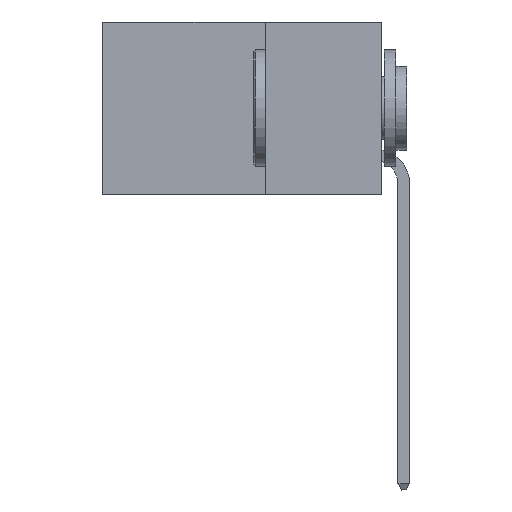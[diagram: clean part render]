
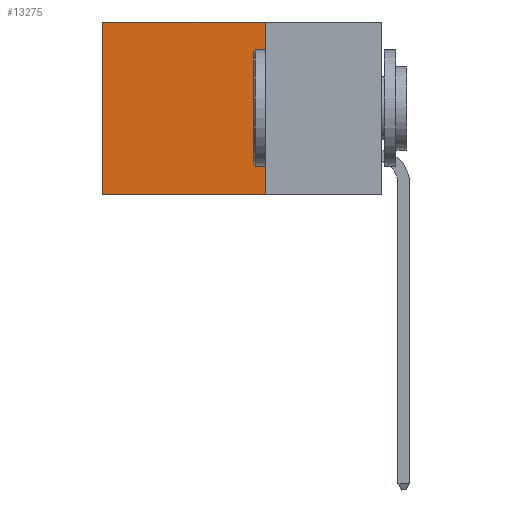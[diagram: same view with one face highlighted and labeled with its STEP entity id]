
A CAD part, left-side view. The second image highlights one B-rep face of the part: STEP entity #13275.
In plain terms, the highlighted planar face has unit normal (-1, 0, 0).
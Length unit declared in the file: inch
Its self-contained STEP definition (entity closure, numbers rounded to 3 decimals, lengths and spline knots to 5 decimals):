
#234 = DIRECTION ( 'NONE',  ( 0., 0., -1. ) ) ;
#1116 = CARTESIAN_POINT ( 'NONE',  ( 0.2875, 0.25, 0. ) ) ;
#3509 = AXIS2_PLACEMENT_3D ( 'NONE', #12520, #12021, #234 ) ;
#4520 = ORIENTED_EDGE ( 'NONE', *, *, #38850, .F. ) ;
#5057 = VERTEX_POINT ( 'NONE', #36150 ) ;
#5293 = CARTESIAN_POINT ( 'NONE',  ( 0.2875, 0.25, -0.37 ) ) ;
#5307 = VECTOR ( 'NONE', #11390, 39.37008 ) ;
#5490 = LINE ( 'NONE', #24578, #9297 ) ;
#6657 = ORIENTED_EDGE ( 'NONE', *, *, #25277, .F. ) ;
#6830 = EDGE_LOOP ( 'NONE', ( #22194, #4520, #6657, #36338 ) ) ;
#9297 = VECTOR ( 'NONE', #13358, 39.37008 ) ;
#11390 = DIRECTION ( 'NONE',  ( 0., 1., 0. ) ) ;
#12021 = DIRECTION ( 'NONE',  ( 1., 0., 0. ) ) ;
#12178 = FACE_OUTER_BOUND ( 'NONE', #6830, .T. ) ;
#12520 = CARTESIAN_POINT ( 'NONE',  ( 0.2875, 0.25, 0. ) ) ;
#13275 = ADVANCED_FACE ( 'NONE', ( #12178 ), #33258, .F. ) ;
#13325 = LINE ( 'NONE', #5293, #5307 ) ;
#13358 = DIRECTION ( 'NONE',  ( 0., 0., -1. ) ) ;
#14139 = DIRECTION ( 'NONE',  ( 0., 1., 0. ) ) ;
#14251 = VECTOR ( 'NONE', #25146, 39.37008 ) ;
#20181 = VERTEX_POINT ( 'NONE', #28641 ) ;
#21384 = LINE ( 'NONE', #26181, #26570 ) ;
#22194 = ORIENTED_EDGE ( 'NONE', *, *, #34258, .T. ) ;
#24578 = CARTESIAN_POINT ( 'NONE',  ( 0.2875, 0.6, 0. ) ) ;
#25146 = DIRECTION ( 'NONE',  ( 0., 0., -1. ) ) ;
#25277 = EDGE_CURVE ( 'NONE', #5057, #20181, #32249, .T. ) ;
#26181 = CARTESIAN_POINT ( 'NONE',  ( 0.2875, 0.25, 0. ) ) ;
#26570 = VECTOR ( 'NONE', #14139, 39.37008 ) ;
#28641 = CARTESIAN_POINT ( 'NONE',  ( 0.2875, 0.25, -0.37 ) ) ;
#30964 = EDGE_CURVE ( 'NONE', #5057, #31340, #21384, .T. ) ;
#31340 = VERTEX_POINT ( 'NONE', #36558 ) ;
#32249 = LINE ( 'NONE', #1116, #14251 ) ;
#33258 = PLANE ( 'NONE',  #3509 ) ;
#34258 = EDGE_CURVE ( 'NONE', #31340, #39076, #5490, .T. ) ;
#36150 = CARTESIAN_POINT ( 'NONE',  ( 0.2875, 0.25, 0. ) ) ;
#36186 = CARTESIAN_POINT ( 'NONE',  ( 0.2875, 0.6, -0.37 ) ) ;
#36338 = ORIENTED_EDGE ( 'NONE', *, *, #30964, .T. ) ;
#36558 = CARTESIAN_POINT ( 'NONE',  ( 0.2875, 0.6, 0. ) ) ;
#38850 = EDGE_CURVE ( 'NONE', #20181, #39076, #13325, .T. ) ;
#39076 = VERTEX_POINT ( 'NONE', #36186 ) ;
